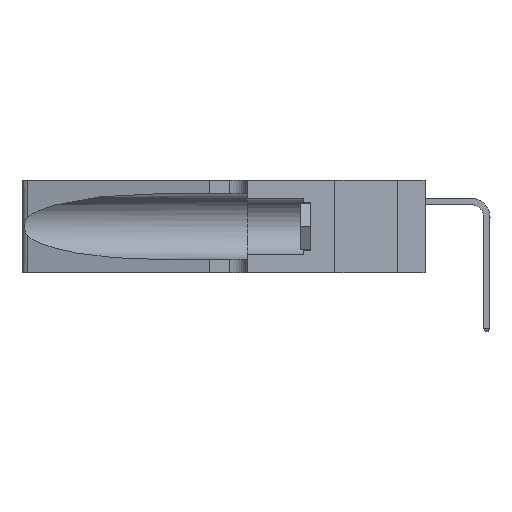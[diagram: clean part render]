
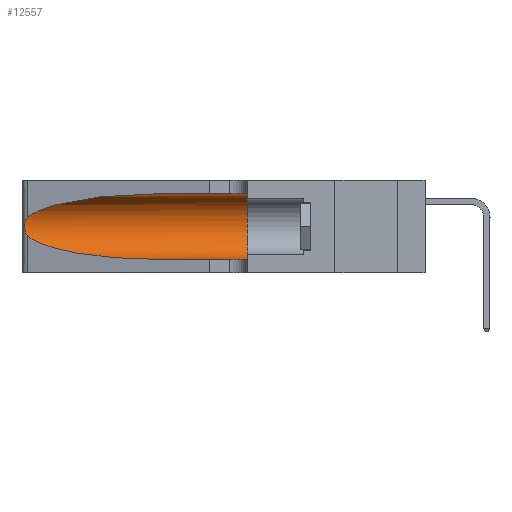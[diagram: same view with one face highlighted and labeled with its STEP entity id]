
A CAD part, left-side view. The second image highlights one B-rep face of the part: STEP entity #12557.
In plain terms, the highlighted cylindrical face has radius 3.308 mm (diameter 6.617 mm), a partial arc.
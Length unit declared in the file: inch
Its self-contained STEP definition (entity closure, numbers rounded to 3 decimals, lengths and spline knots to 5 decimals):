
#91 = VERTEX_POINT ( 'NONE', #6390 ) ;
#1192 = VERTEX_POINT ( 'NONE', #11662 ) ;
#1297 = CARTESIAN_POINT ( 'NONE',  ( 0.1305, 0.35, 0.05475 ) ) ;
#1516 = DIRECTION ( 'NONE',  ( 0., 1., 0. ) ) ;
#1699 = CARTESIAN_POINT ( 'NONE',  ( 0.25487, 1.22718, 0.14631 ) ) ;
#2120 = CARTESIAN_POINT ( 'NONE',  ( 0.25787, 1.23484, 0.2124 ) ) ;
#2569 = CARTESIAN_POINT ( 'NONE',  ( 0.1305, 0.72297, 0.31525 ) ) ;
#2639 = LINE ( 'NONE', #7944, #14502 ) ;
#3496 = VERTEX_POINT ( 'NONE', #13308 ) ;
#3582 = CARTESIAN_POINT ( 'NONE',  ( 0.26018, 1.23835, 0.19895 ) ) ;
#3724 = CARTESIAN_POINT ( 'NONE',  ( 0.1305, 1.61858, 0.05475 ) ) ;
#3865 = EDGE_CURVE ( 'NONE', #3496, #15307, #9104, .T. ) ;
#4633 = CARTESIAN_POINT ( 'NONE',  ( 0.1305, 0.72297, 0.05475 ) ) ;
#4987 = ORIENTED_EDGE ( 'NONE', *, *, #11334, .F. ) ;
#5047 = CARTESIAN_POINT ( 'NONE',  ( 0.26075, 1.23896, 0.178 ) ) ;
#5175 = EDGE_LOOP ( 'NONE', ( #11555, #10655, #13371, #10466, #11456, #4987 ) ) ;
#5241 = CARTESIAN_POINT ( 'NONE',  ( 0.18966, 0.96281, 0.31525 ) ) ;
#5293 = AXIS2_PLACEMENT_3D ( 'NONE', #10333, #1516, #11856 ) ;
#5928 = EDGE_CURVE ( 'NONE', #1192, #3496, #8633, .T. ) ;
#6205 = EDGE_CURVE ( 'NONE', #10348, #10816, #18356, .T. ) ;
#6390 = CARTESIAN_POINT ( 'NONE',  ( 0.1305, 0.35, 0.31525 ) ) ;
#6486 = CARTESIAN_POINT ( 'NONE',  ( 0.25555, 1.22994, 0.2215 ) ) ;
#6552 = CARTESIAN_POINT ( 'NONE',  ( 0.25856, 1.23593, 0.16098 ) ) ;
#7006 = FACE_OUTER_BOUND ( 'NONE', #5175, .T. ) ;
#7711 = DIRECTION ( 'NONE',  ( 0., -1., 0. ) ) ;
#7827 = EDGE_CURVE ( 'NONE', #91, #15307, #18507, .T. ) ;
#7944 = CARTESIAN_POINT ( 'NONE',  ( 0.1305, 1.61858, 0.31525 ) ) ;
#8031 = CARTESIAN_POINT ( 'NONE',  ( 0.25639, 1.23186, 0.15144 ) ) ;
#8241 = CARTESIAN_POINT ( 'NONE',  ( 0.1305, 0.72297, 0.31525 ) ) ;
#8633 =( BOUNDED_CURVE ( )  B_SPLINE_CURVE ( 3, ( #1699, #12058, #13569, #4633 ),
 .UNSPECIFIED., .F., .F. ) 
 B_SPLINE_CURVE_WITH_KNOTS ( ( 4, 4 ),
 ( 3.44316, 4.71239 ),
 .UNSPECIFIED. ) 
 CURVE ( )  GEOMETRIC_REPRESENTATION_ITEM ( )  RATIONAL_B_SPLINE_CURVE ( ( 1., 0.87, 0.87, 1. ) ) 
 REPRESENTATION_ITEM ( '' )  );
#8637 = VECTOR ( 'NONE', #11170, 39.37008 ) ;
#9104 = LINE ( 'NONE', #3724, #8637 ) ;
#9440 = DIRECTION ( 'NONE',  ( 0., -1., 0. ) ) ;
#9514 = CARTESIAN_POINT ( 'NONE',  ( 0.25487, 1.22718, 0.22369 ) ) ;
#9535 = CARTESIAN_POINT ( 'NONE',  ( 0.25487, 1.22718, 0.14631 ) ) ;
#10333 = CARTESIAN_POINT ( 'NONE',  ( 0.1305, 0.35, 0.185 ) ) ;
#10348 = VERTEX_POINT ( 'NONE', #2569 ) ;
#10432 = B_SPLINE_CURVE_WITH_KNOTS ( 'NONE', 3,
 ( #10890, #6486, #10960, #2120, #12499, #3582, #14018, #5047, #15498, #6552, #16952, #8031, #18411, #9535 ),
 .UNSPECIFIED., .F., .F.,
 ( 4, 2, 2, 2, 2, 2, 4 ),
 ( 0., 0.00027, 0.00053, 0.00107, 0.0016, 0.00187, 0.00214 ),
 .UNSPECIFIED. ) ;
#10466 = ORIENTED_EDGE ( 'NONE', *, *, #3865, .T. ) ;
#10655 = ORIENTED_EDGE ( 'NONE', *, *, #13725, .T. ) ;
#10680 = CARTESIAN_POINT ( 'NONE',  ( 0.1305, 1.61858, 0.185 ) ) ;
#10816 = VERTEX_POINT ( 'NONE', #9514 ) ;
#10890 = CARTESIAN_POINT ( 'NONE',  ( 0.25487, 1.22718, 0.22369 ) ) ;
#10960 = CARTESIAN_POINT ( 'NONE',  ( 0.25639, 1.23184, 0.21858 ) ) ;
#11170 = DIRECTION ( 'NONE',  ( 0., -1., 0. ) ) ;
#11334 = EDGE_CURVE ( 'NONE', #10348, #91, #2639, .T. ) ;
#11456 = ORIENTED_EDGE ( 'NONE', *, *, #7827, .F. ) ;
#11555 = ORIENTED_EDGE ( 'NONE', *, *, #6205, .T. ) ;
#11662 = CARTESIAN_POINT ( 'NONE',  ( 0.25487, 1.22718, 0.14631 ) ) ;
#11856 = DIRECTION ( 'NONE',  ( 0., 0., 1. ) ) ;
#12058 = CARTESIAN_POINT ( 'NONE',  ( 0.2373, 1.15595, 0.08982 ) ) ;
#12499 = CARTESIAN_POINT ( 'NONE',  ( 0.25854, 1.2359, 0.20912 ) ) ;
#12557 = ADVANCED_FACE ( 'NONE', ( #7006 ), #17452, .F. ) ;
#12703 = CARTESIAN_POINT ( 'NONE',  ( 0.2373, 1.15595, 0.28018 ) ) ;
#13308 = CARTESIAN_POINT ( 'NONE',  ( 0.1305, 0.72297, 0.05475 ) ) ;
#13371 = ORIENTED_EDGE ( 'NONE', *, *, #5928, .T. ) ;
#13569 = CARTESIAN_POINT ( 'NONE',  ( 0.18966, 0.96281, 0.05475 ) ) ;
#13725 = EDGE_CURVE ( 'NONE', #10816, #1192, #10432, .T. ) ;
#14018 = CARTESIAN_POINT ( 'NONE',  ( 0.26075, 1.23896, 0.19203 ) ) ;
#14502 = VECTOR ( 'NONE', #9440, 39.37008 ) ;
#15026 = AXIS2_PLACEMENT_3D ( 'NONE', #10680, #7711, #15246 ) ;
#15246 = DIRECTION ( 'NONE',  ( 0., 0., -1. ) ) ;
#15307 = VERTEX_POINT ( 'NONE', #1297 ) ;
#15498 = CARTESIAN_POINT ( 'NONE',  ( 0.26017, 1.23833, 0.17102 ) ) ;
#16952 = CARTESIAN_POINT ( 'NONE',  ( 0.25789, 1.23486, 0.15765 ) ) ;
#17452 = CYLINDRICAL_SURFACE ( 'NONE', #15026, 0.13025 ) ;
#18356 =( BOUNDED_CURVE ( )  B_SPLINE_CURVE ( 3, ( #8241, #5241, #12703, #18608 ),
 .UNSPECIFIED., .F., .T. ) 
 B_SPLINE_CURVE_WITH_KNOTS ( ( 4, 4 ),
 ( 1.5708, 2.84003 ),
 .UNSPECIFIED. ) 
 CURVE ( )  GEOMETRIC_REPRESENTATION_ITEM ( )  RATIONAL_B_SPLINE_CURVE ( ( 1., 0.87, 0.87, 1. ) ) 
 REPRESENTATION_ITEM ( '' )  );
#18411 = CARTESIAN_POINT ( 'NONE',  ( 0.25555, 1.22993, 0.14849 ) ) ;
#18507 = CIRCLE ( 'NONE', #5293, 0.13025 ) ;
#18608 = CARTESIAN_POINT ( 'NONE',  ( 0.25487, 1.22718, 0.22369 ) ) ;
